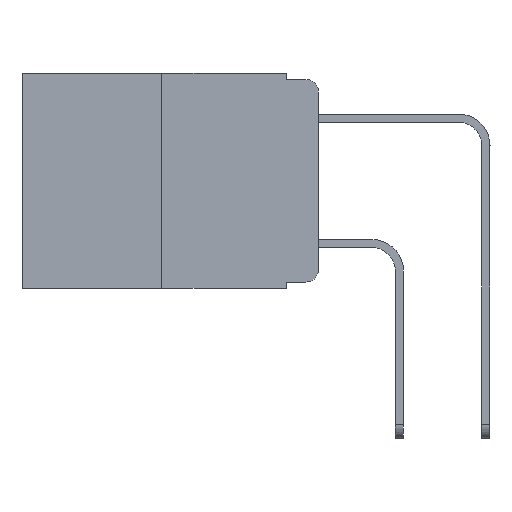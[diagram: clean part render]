
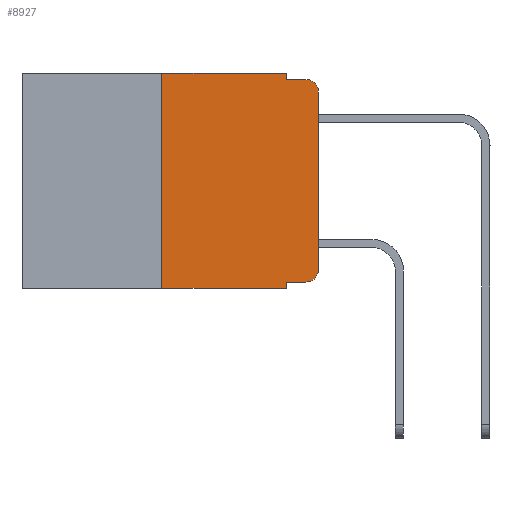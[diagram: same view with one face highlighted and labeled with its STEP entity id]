
A CAD part, left-side view. The second image highlights one B-rep face of the part: STEP entity #8927.
In plain terms, the highlighted planar face has unit normal (-1, 0, 0).
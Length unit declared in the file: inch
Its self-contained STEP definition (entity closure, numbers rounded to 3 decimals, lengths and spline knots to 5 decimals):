
#5 = CARTESIAN_POINT ( 'NONE',  ( 0., 0.051, -0.01 ) ) ;
#76 = CARTESIAN_POINT ( 'NONE',  ( 0., 0.051, -0.333 ) ) ;
#181 = EDGE_CURVE ( 'NONE', #915, #7464, #8750, .T. ) ;
#302 = VERTEX_POINT ( 'NONE', #3111 ) ;
#307 = AXIS2_PLACEMENT_3D ( 'NONE', #4935, #9083, #10871 ) ;
#729 = ORIENTED_EDGE ( 'NONE', *, *, #181, .T. ) ;
#848 = LINE ( 'NONE', #2838, #10348 ) ;
#874 = CARTESIAN_POINT ( 'NONE',  ( 0., 0.473, 0. ) ) ;
#915 = VERTEX_POINT ( 'NONE', #8439 ) ;
#1097 = LINE ( 'NONE', #10720, #10874 ) ;
#1183 = DIRECTION ( 'NONE',  ( 0., 0., 1. ) ) ;
#1210 = ORIENTED_EDGE ( 'NONE', *, *, #5407, .T. ) ;
#1484 = CIRCLE ( 'NONE', #7201, 0.02 ) ;
#1716 = DIRECTION ( 'NONE',  ( 1., 0., 0. ) ) ;
#1776 = VERTEX_POINT ( 'NONE', #76 ) ;
#1862 = EDGE_CURVE ( 'NONE', #1776, #915, #848, .T. ) ;
#1903 = VECTOR ( 'NONE', #7952, 39.37008 ) ;
#1932 = EDGE_CURVE ( 'NONE', #8234, #6264, #8321, .T. ) ;
#2294 = CARTESIAN_POINT ( 'NONE',  ( 0., 0.25, 0. ) ) ;
#2468 = ORIENTED_EDGE ( 'NONE', *, *, #8218, .T. ) ;
#2500 = VECTOR ( 'NONE', #5646, 39.37008 ) ;
#2621 = CARTESIAN_POINT ( 'NONE',  ( 0., 0.02, -0.01 ) ) ;
#2838 = CARTESIAN_POINT ( 'NONE',  ( 0., 0.051, -0.333 ) ) ;
#3106 = DIRECTION ( 'NONE',  ( 0., 0., 1. ) ) ;
#3111 = CARTESIAN_POINT ( 'NONE',  ( 0., 0.051, 0. ) ) ;
#3596 = ORIENTED_EDGE ( 'NONE', *, *, #9343, .T. ) ;
#3619 = VECTOR ( 'NONE', #10397, 39.37008 ) ;
#3622 = ORIENTED_EDGE ( 'NONE', *, *, #9213, .F. ) ;
#3662 = DIRECTION ( 'NONE',  ( 0., -1., 0. ) ) ;
#4011 = CARTESIAN_POINT ( 'NONE',  ( 0., 0.051, -0.01 ) ) ;
#4051 = VERTEX_POINT ( 'NONE', #2621 ) ;
#4283 = DIRECTION ( 'NONE',  ( 0., 0., -1. ) ) ;
#4627 = CARTESIAN_POINT ( 'NONE',  ( 0., 0.051, 0. ) ) ;
#4935 = CARTESIAN_POINT ( 'NONE',  ( 0., 0.02, -0.313 ) ) ;
#5081 = DIRECTION ( 'NONE',  ( -1., 0., 0. ) ) ;
#5400 = ORIENTED_EDGE ( 'NONE', *, *, #7888, .F. ) ;
#5407 = EDGE_CURVE ( 'NONE', #8234, #6133, #10114, .T. ) ;
#5483 = LINE ( 'NONE', #7838, #1903 ) ;
#5584 = DIRECTION ( 'NONE',  ( 0., 0., -1. ) ) ;
#5646 = DIRECTION ( 'NONE',  ( 0., -1., 0. ) ) ;
#5886 = EDGE_CURVE ( 'NONE', #6249, #4051, #9818, .T. ) ;
#6085 = PLANE ( 'NONE',  #6759 ) ;
#6133 = VERTEX_POINT ( 'NONE', #8757 ) ;
#6249 = VERTEX_POINT ( 'NONE', #4011 ) ;
#6264 = VERTEX_POINT ( 'NONE', #2294 ) ;
#6757 = LINE ( 'NONE', #7470, #8637 ) ;
#6759 = AXIS2_PLACEMENT_3D ( 'NONE', #874, #1716, #4283 ) ;
#6788 = CARTESIAN_POINT ( 'NONE',  ( 0., 0.02, -0.03 ) ) ;
#7110 = ORIENTED_EDGE ( 'NONE', *, *, #1862, .T. ) ;
#7201 = AXIS2_PLACEMENT_3D ( 'NONE', #6788, #5081, #10157 ) ;
#7464 = VERTEX_POINT ( 'NONE', #8255 ) ;
#7468 = ORIENTED_EDGE ( 'NONE', *, *, #1932, .F. ) ;
#7470 = CARTESIAN_POINT ( 'NONE',  ( 0., 0., 0. ) ) ;
#7785 = VECTOR ( 'NONE', #1183, 39.37008 ) ;
#7826 = EDGE_CURVE ( 'NONE', #6264, #302, #5483, .T. ) ;
#7838 = CARTESIAN_POINT ( 'NONE',  ( 0., 0.473, 0. ) ) ;
#7888 = EDGE_CURVE ( 'NONE', #302, #6249, #1097, .T. ) ;
#7952 = DIRECTION ( 'NONE',  ( 0., -1., 0. ) ) ;
#8110 = CARTESIAN_POINT ( 'NONE',  ( 0., 0.25, 0. ) ) ;
#8218 = EDGE_CURVE ( 'NONE', #9909, #4051, #1484, .T. ) ;
#8234 = VERTEX_POINT ( 'NONE', #8459 ) ;
#8255 = CARTESIAN_POINT ( 'NONE',  ( 0., 0., -0.313 ) ) ;
#8321 = LINE ( 'NONE', #8110, #7785 ) ;
#8407 = VECTOR ( 'NONE', #5584, 39.37008 ) ;
#8411 = FACE_OUTER_BOUND ( 'NONE', #9508, .T. ) ;
#8439 = CARTESIAN_POINT ( 'NONE',  ( 0., 0.02, -0.333 ) ) ;
#8459 = CARTESIAN_POINT ( 'NONE',  ( 0., 0.25, -0.343 ) ) ;
#8637 = VECTOR ( 'NONE', #3106, 39.37008 ) ;
#8750 = CIRCLE ( 'NONE', #307, 0.02 ) ;
#8757 = CARTESIAN_POINT ( 'NONE',  ( 0., 0.051, -0.343 ) ) ;
#8927 = ADVANCED_FACE ( 'NONE', ( #8411 ), #6085, .F. ) ;
#8958 = CARTESIAN_POINT ( 'NONE',  ( 0., 0., -0.03 ) ) ;
#9083 = DIRECTION ( 'NONE',  ( -1., 0., 0. ) ) ;
#9213 = EDGE_CURVE ( 'NONE', #1776, #6133, #10703, .T. ) ;
#9240 = ORIENTED_EDGE ( 'NONE', *, *, #7826, .F. ) ;
#9343 = EDGE_CURVE ( 'NONE', #7464, #9909, #6757, .T. ) ;
#9508 = EDGE_LOOP ( 'NONE', ( #3596, #2468, #9845, #5400, #9240, #7468, #1210, #3622, #7110, #729 ) ) ;
#9818 = LINE ( 'NONE', #5, #3619 ) ;
#9822 = DIRECTION ( 'NONE',  ( 0., 0., -1. ) ) ;
#9845 = ORIENTED_EDGE ( 'NONE', *, *, #5886, .F. ) ;
#9909 = VERTEX_POINT ( 'NONE', #8958 ) ;
#10114 = LINE ( 'NONE', #10777, #2500 ) ;
#10157 = DIRECTION ( 'NONE',  ( 0., 0., -1. ) ) ;
#10348 = VECTOR ( 'NONE', #3662, 39.37008 ) ;
#10397 = DIRECTION ( 'NONE',  ( 0., -1., 0. ) ) ;
#10703 = LINE ( 'NONE', #4627, #8407 ) ;
#10720 = CARTESIAN_POINT ( 'NONE',  ( 0., 0.051, 0. ) ) ;
#10777 = CARTESIAN_POINT ( 'NONE',  ( 0., 0.473, -0.343 ) ) ;
#10871 = DIRECTION ( 'NONE',  ( 0., 0., -1. ) ) ;
#10874 = VECTOR ( 'NONE', #9822, 39.37008 ) ;
